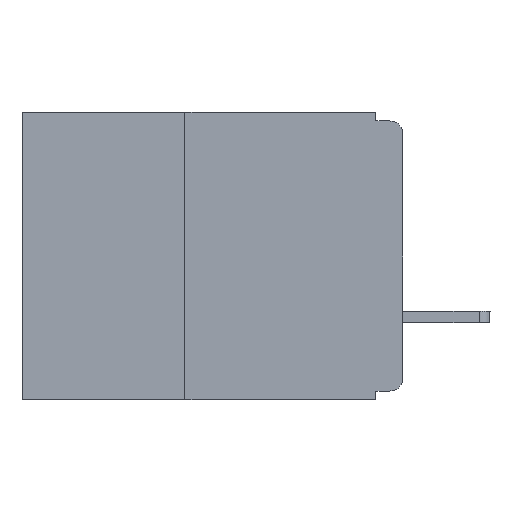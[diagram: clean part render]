
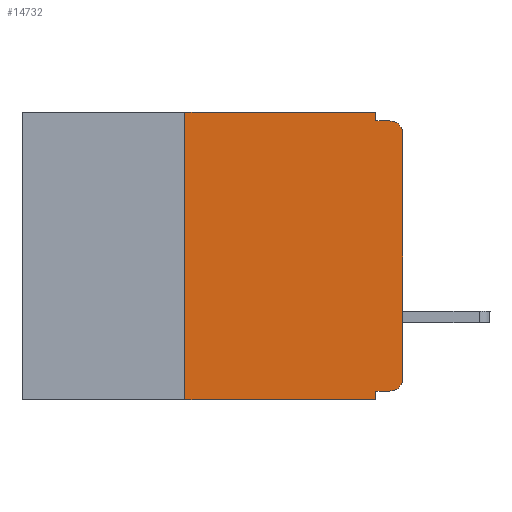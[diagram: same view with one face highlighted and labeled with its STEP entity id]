
A CAD part, left-side view. The second image highlights one B-rep face of the part: STEP entity #14732.
In plain terms, the highlighted planar face has unit normal (-1, 0, 0).
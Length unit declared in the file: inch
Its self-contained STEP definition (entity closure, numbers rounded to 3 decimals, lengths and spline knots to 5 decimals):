
#46 = VECTOR ( 'NONE', #9014, 39.37008 ) ;
#329 = CARTESIAN_POINT ( 'NONE',  ( 0., 0.031, -0.33 ) ) ;
#493 = CARTESIAN_POINT ( 'NONE',  ( 0., 0.031, -0.32 ) ) ;
#505 = AXIS2_PLACEMENT_3D ( 'NONE', #5273, #1705, #11074 ) ;
#523 = CIRCLE ( 'NONE', #12184, 0.015 ) ;
#536 = CARTESIAN_POINT ( 'NONE',  ( 0., 0., -0.305 ) ) ;
#569 = DIRECTION ( 'NONE',  ( 0., -1., 0. ) ) ;
#928 = EDGE_CURVE ( 'NONE', #12525, #11043, #8517, .T. ) ;
#1098 = VERTEX_POINT ( 'NONE', #12210 ) ;
#1242 = VERTEX_POINT ( 'NONE', #2304 ) ;
#1308 = EDGE_CURVE ( 'NONE', #11043, #11346, #523, .T. ) ;
#1705 = DIRECTION ( 'NONE',  ( 1., 0., 0. ) ) ;
#1913 = LINE ( 'NONE', #5743, #4056 ) ;
#2195 = DIRECTION ( 'NONE',  ( 0., 0., -1. ) ) ;
#2217 = EDGE_CURVE ( 'NONE', #4730, #1242, #11054, .T. ) ;
#2304 = CARTESIAN_POINT ( 'NONE',  ( 0., 0.031, -0.33 ) ) ;
#2382 = CARTESIAN_POINT ( 'NONE',  ( 0., 0., 0. ) ) ;
#2411 = LINE ( 'NONE', #5093, #2763 ) ;
#2661 = CARTESIAN_POINT ( 'NONE',  ( 0., 0.015, -0.32 ) ) ;
#2679 = CARTESIAN_POINT ( 'NONE',  ( 0., 0., -0.01 ) ) ;
#2763 = VECTOR ( 'NONE', #8627, 39.37008 ) ;
#2772 = CARTESIAN_POINT ( 'NONE',  ( 0., 0.015, -0.01 ) ) ;
#2878 = ORIENTED_EDGE ( 'NONE', *, *, #928, .T. ) ;
#3149 = EDGE_CURVE ( 'NONE', #3632, #11346, #8815, .T. ) ;
#3209 = CARTESIAN_POINT ( 'NONE',  ( 0., 0.437, -0.33 ) ) ;
#3632 = VERTEX_POINT ( 'NONE', #11616 ) ;
#4056 = VECTOR ( 'NONE', #4622, 39.37008 ) ;
#4202 = CARTESIAN_POINT ( 'NONE',  ( 0., 0.25, -0.33 ) ) ;
#4365 = LINE ( 'NONE', #11252, #46 ) ;
#4622 = DIRECTION ( 'NONE',  ( 0., 1., 0. ) ) ;
#4730 = VERTEX_POINT ( 'NONE', #493 ) ;
#4967 = VECTOR ( 'NONE', #5448, 39.37008 ) ;
#5093 = CARTESIAN_POINT ( 'NONE',  ( 0., 0.25, -0.33 ) ) ;
#5168 = VERTEX_POINT ( 'NONE', #4202 ) ;
#5273 = CARTESIAN_POINT ( 'NONE',  ( 0., 0.437, 0. ) ) ;
#5322 = VECTOR ( 'NONE', #569, 39.37008 ) ;
#5448 = DIRECTION ( 'NONE',  ( 0., -1., 0. ) ) ;
#5726 = DIRECTION ( 'NONE',  ( 0., 0., 1. ) ) ;
#5743 = CARTESIAN_POINT ( 'NONE',  ( 0., 0., -0.32 ) ) ;
#5944 = DIRECTION ( 'NONE',  ( 0., 0., -1. ) ) ;
#6246 = CARTESIAN_POINT ( 'NONE',  ( 0., 0.015, -0.305 ) ) ;
#6285 = VERTEX_POINT ( 'NONE', #8011 ) ;
#6358 = DIRECTION ( 'NONE',  ( -1., 0., 0. ) ) ;
#6458 = ORIENTED_EDGE ( 'NONE', *, *, #12490, .T. ) ;
#6738 = EDGE_LOOP ( 'NONE', ( #2878, #10083, #13971, #10597, #11757, #9813, #8988, #10357, #9754, #6458 ) ) ;
#6992 = FACE_OUTER_BOUND ( 'NONE', #6738, .T. ) ;
#7209 = VECTOR ( 'NONE', #5944, 39.37008 ) ;
#7572 = EDGE_CURVE ( 'NONE', #6285, #3632, #4365, .T. ) ;
#7911 = EDGE_CURVE ( 'NONE', #5168, #1098, #2411, .T. ) ;
#8011 = CARTESIAN_POINT ( 'NONE',  ( 0., 0.031, 0. ) ) ;
#8125 = DIRECTION ( 'NONE',  ( -1., 0., 0. ) ) ;
#8345 = AXIS2_PLACEMENT_3D ( 'NONE', #6246, #6358, #13389 ) ;
#8517 = LINE ( 'NONE', #2382, #8891 ) ;
#8627 = DIRECTION ( 'NONE',  ( 0., 0., 1. ) ) ;
#8796 = CARTESIAN_POINT ( 'NONE',  ( 0., 0., -0.025 ) ) ;
#8815 = LINE ( 'NONE', #2679, #5322 ) ;
#8891 = VECTOR ( 'NONE', #5726, 39.37008 ) ;
#8988 = ORIENTED_EDGE ( 'NONE', *, *, #14382, .T. ) ;
#9014 = DIRECTION ( 'NONE',  ( 0., 0., -1. ) ) ;
#9741 = LINE ( 'NONE', #3209, #4967 ) ;
#9754 = ORIENTED_EDGE ( 'NONE', *, *, #14976, .F. ) ;
#9813 = ORIENTED_EDGE ( 'NONE', *, *, #7911, .F. ) ;
#9903 = CARTESIAN_POINT ( 'NONE',  ( 0., 0.437, 0. ) ) ;
#9996 = CIRCLE ( 'NONE', #8345, 0.015 ) ;
#10083 = ORIENTED_EDGE ( 'NONE', *, *, #1308, .T. ) ;
#10357 = ORIENTED_EDGE ( 'NONE', *, *, #2217, .F. ) ;
#10476 = CARTESIAN_POINT ( 'NONE',  ( 0., 0.015, -0.025 ) ) ;
#10597 = ORIENTED_EDGE ( 'NONE', *, *, #7572, .F. ) ;
#10731 = LINE ( 'NONE', #9903, #12374 ) ;
#11021 = DIRECTION ( 'NONE',  ( 0., -1., 0. ) ) ;
#11043 = VERTEX_POINT ( 'NONE', #8796 ) ;
#11054 = LINE ( 'NONE', #329, #7209 ) ;
#11074 = DIRECTION ( 'NONE',  ( 0., 0., -1. ) ) ;
#11252 = CARTESIAN_POINT ( 'NONE',  ( 0., 0.031, 0. ) ) ;
#11346 = VERTEX_POINT ( 'NONE', #2772 ) ;
#11616 = CARTESIAN_POINT ( 'NONE',  ( 0., 0.031, -0.01 ) ) ;
#11757 = ORIENTED_EDGE ( 'NONE', *, *, #12509, .F. ) ;
#12184 = AXIS2_PLACEMENT_3D ( 'NONE', #10476, #8125, #2195 ) ;
#12210 = CARTESIAN_POINT ( 'NONE',  ( 0., 0.25, 0. ) ) ;
#12374 = VECTOR ( 'NONE', #11021, 39.37008 ) ;
#12490 = EDGE_CURVE ( 'NONE', #13455, #12525, #9996, .T. ) ;
#12509 = EDGE_CURVE ( 'NONE', #1098, #6285, #10731, .T. ) ;
#12525 = VERTEX_POINT ( 'NONE', #536 ) ;
#13389 = DIRECTION ( 'NONE',  ( 0., 0., -1. ) ) ;
#13455 = VERTEX_POINT ( 'NONE', #2661 ) ;
#13564 = PLANE ( 'NONE',  #505 ) ;
#13971 = ORIENTED_EDGE ( 'NONE', *, *, #3149, .F. ) ;
#14382 = EDGE_CURVE ( 'NONE', #5168, #1242, #9741, .T. ) ;
#14732 = ADVANCED_FACE ( 'NONE', ( #6992 ), #13564, .F. ) ;
#14976 = EDGE_CURVE ( 'NONE', #13455, #4730, #1913, .T. ) ;
